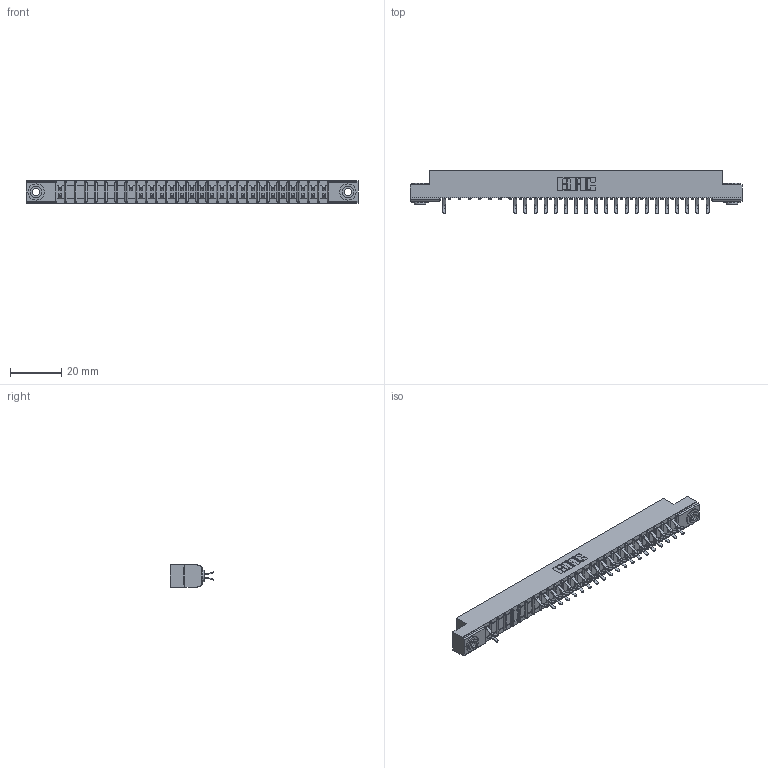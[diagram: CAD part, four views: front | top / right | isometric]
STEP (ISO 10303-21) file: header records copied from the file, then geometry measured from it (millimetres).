
FILE_DESCRIPTION (( 'STEP AP203' ), '1' );
FILE_NAME ('307-054-556-203.STEP', '2018-08-06T06:12:35', ( '' ), ( '' ), 'SwSTEP 2.0', 'SolidWorks 2016', '' );
FILE_SCHEMA (( 'CONFIG_CONTROL_DESIGN' ));
Length unit declared in the file: inch
Products named in the file (4): 307 Part_.156 Dia Mounting Holes; 307-290-001_556; 345-250-002_345-250-002-102; 307-054-556-203
Assembly tree (44 placements, depth 2):
  307-054-556-203
    307 Part_.156 Dia Mounting Holes
    307-290-001_556  x41
    345-250-002_345-250-002-102  x2
Bounding box: 130 x 16.97 x 8.71 mm (x, y, z)
Volume: 8328.2 mm3; surface area: 14182.7 mm2
Topology: 44 solids, 44 shells, 2378 faces, 6673 edges, 4314 vertices
Faces by surface type: plane 1525, cylinder 789, sphere 56, cone 8
Entity records: 26613 total; most frequent: CARTESIAN_POINT 4395, ORIENTED_EDGE 4358, DIRECTION 4313, EDGE_CURVE 2179, VECTOR 1657, LINE 1657, VERTEX_POINT 1410, AXIS2_PLACEMENT_3D 1328
